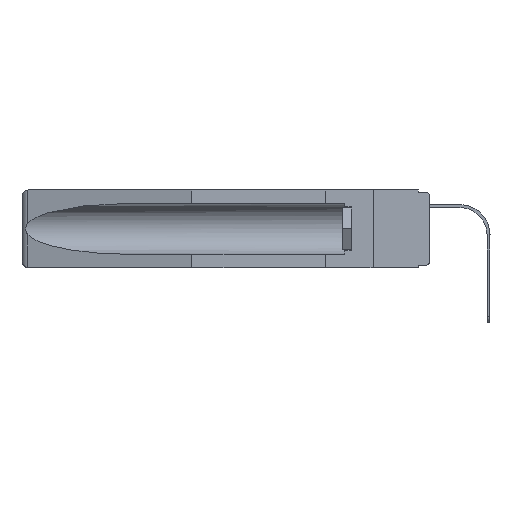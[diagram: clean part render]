
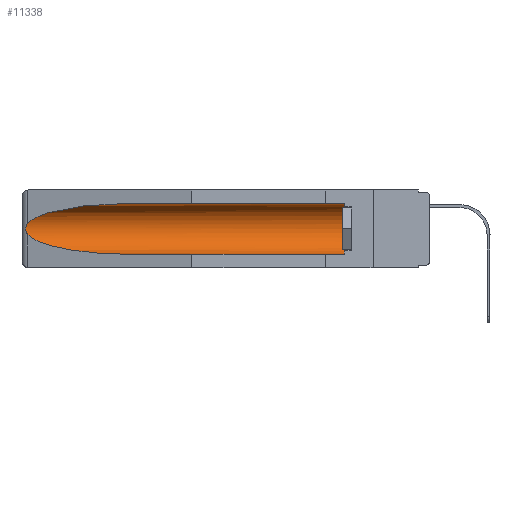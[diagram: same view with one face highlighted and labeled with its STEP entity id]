
A CAD part, left-side view. The second image highlights one B-rep face of the part: STEP entity #11338.
In plain terms, the highlighted cylindrical face has radius 2.857 mm (diameter 5.715 mm), a partial arc.
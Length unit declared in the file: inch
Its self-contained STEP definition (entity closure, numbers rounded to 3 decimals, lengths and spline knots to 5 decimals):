
#550 = EDGE_LOOP ( 'NONE', ( #24574, #18355, #9766, #16746, #15349, #6919 ) ) ;
#585 = CARTESIAN_POINT ( 'NONE',  ( 0.21114, 1.30732, -0.284 ) ) ;
#744 = DIRECTION ( 'NONE',  ( 0., 1., 0. ) ) ;
#991 = DIRECTION ( 'NONE',  ( 0., -1., 0. ) ) ;
#1263 = AXIS2_PLACEMENT_3D ( 'NONE', #24435, #22390, #2885 ) ;
#2885 = DIRECTION ( 'NONE',  ( 0., 0., 1. ) ) ;
#3160 = CARTESIAN_POINT ( 'NONE',  ( 0.2675, 1.53308, -0.17534 ) ) ;
#3287 = CARTESIAN_POINT ( 'NONE',  ( 0.26597, 1.5296, -0.19026 ) ) ;
#4566 = EDGE_CURVE ( 'NONE', #14290, #7133, #9843, .T. ) ;
#4671 = VERTEX_POINT ( 'NONE', #20564 ) ;
#5633 = CARTESIAN_POINT ( 'NONE',  ( 0.155, -0.30754, -0.059 ) ) ;
#6863 = AXIS2_PLACEMENT_3D ( 'NONE', #12802, #991, #18305 ) ;
#6919 = ORIENTED_EDGE ( 'NONE', *, *, #4566, .T. ) ;
#7133 = VERTEX_POINT ( 'NONE', #23824 ) ;
#7263 = EDGE_CURVE ( 'NONE', #15653, #7328, #10865, .T. ) ;
#7293 = EDGE_CURVE ( 'NONE', #15653, #14290, #20357, .T. ) ;
#7328 = VERTEX_POINT ( 'NONE', #12676 ) ;
#7773 = EDGE_CURVE ( 'NONE', #4671, #7328, #22846, .T. ) ;
#8536 = CARTESIAN_POINT ( 'NONE',  ( 0.26537, 1.52718, -0.19328 ) ) ;
#8577 = EDGE_CURVE ( 'NONE', #12557, #4671, #16978, .T. ) ;
#9313 = CARTESIAN_POINT ( 'NONE',  ( 0.2673, 1.5327, -0.16383 ) ) ;
#9766 = ORIENTED_EDGE ( 'NONE', *, *, #7773, .T. ) ;
#9843 = LINE ( 'NONE', #5633, #10423 ) ;
#9967 = DIRECTION ( 'NONE',  ( 0., 1., 0. ) ) ;
#10423 = VECTOR ( 'NONE', #9967, 39.37008 ) ;
#10459 = FACE_OUTER_BOUND ( 'NONE', #550, .T. ) ;
#10865 = LINE ( 'NONE', #16646, #22420 ) ;
#11338 = ADVANCED_FACE ( 'NONE', ( #10459 ), #16618, .F. ) ;
#11370 = CARTESIAN_POINT ( 'NONE',  ( 0.26537, 1.52718, -0.19328 ) ) ;
#12557 = VERTEX_POINT ( 'NONE', #24482 ) ;
#12676 = CARTESIAN_POINT ( 'NONE',  ( 0.155, 1.07973, -0.284 ) ) ;
#12802 = CARTESIAN_POINT ( 'NONE',  ( 0.155, 0.126, -0.1715 ) ) ;
#12920 = CARTESIAN_POINT ( 'NONE',  ( 0.2675, 1.53308, -0.16763 ) ) ;
#14290 = VERTEX_POINT ( 'NONE', #20853 ) ;
#14327 = CARTESIAN_POINT ( 'NONE',  ( 0.155, 1.07973, -0.284 ) ) ;
#14851 = CARTESIAN_POINT ( 'NONE',  ( 0.26654, 1.53092, -0.15636 ) ) ;
#15349 = ORIENTED_EDGE ( 'NONE', *, *, #7293, .T. ) ;
#15653 = VERTEX_POINT ( 'NONE', #22382 ) ;
#15775 = CARTESIAN_POINT ( 'NONE',  ( 0.21114, 1.30732, -0.059 ) ) ;
#16501 = EDGE_CURVE ( 'NONE', #7133, #12557, #17585, .T. ) ;
#16618 = CYLINDRICAL_SURFACE ( 'NONE', #1263, 0.1125 ) ;
#16646 = CARTESIAN_POINT ( 'NONE',  ( 0.155, -0.30754, -0.284 ) ) ;
#16746 = ORIENTED_EDGE ( 'NONE', *, *, #7263, .F. ) ;
#16884 = CARTESIAN_POINT ( 'NONE',  ( 0.2673, 1.53269, -0.17917 ) ) ;
#16978 = B_SPLINE_CURVE_WITH_KNOTS ( 'NONE', 3,
 ( #20725, #18921, #14851, #9313, #12920, #3160, #16884, #17147, #3287, #11370 ),
 .UNSPECIFIED., .F., .F.,
 ( 4, 2, 2, 2, 4 ),
 ( 0., 0.00029, 0.00058, 0.00087, 0.00117 ),
 .UNSPECIFIED. ) ;
#17147 = CARTESIAN_POINT ( 'NONE',  ( 0.26655, 1.53094, -0.18657 ) ) ;
#17585 =( BOUNDED_CURVE ( )  B_SPLINE_CURVE ( 3, ( #25017, #15775, #23336, #23092 ),
 .UNSPECIFIED., .F., .F. ) 
 B_SPLINE_CURVE_WITH_KNOTS ( ( 4, 4 ),
 ( 4.71239, 6.08839 ),
 .UNSPECIFIED. ) 
 CURVE ( )  GEOMETRIC_REPRESENTATION_ITEM ( )  RATIONAL_B_SPLINE_CURVE ( ( 1., 0.848, 0.848, 1. ) ) 
 REPRESENTATION_ITEM ( '' )  );
#18147 = CARTESIAN_POINT ( 'NONE',  ( 0.25451, 1.48313, -0.24835 ) ) ;
#18305 = DIRECTION ( 'NONE',  ( 0., 0., 1. ) ) ;
#18355 = ORIENTED_EDGE ( 'NONE', *, *, #8577, .T. ) ;
#18921 = CARTESIAN_POINT ( 'NONE',  ( 0.26597, 1.52961, -0.15275 ) ) ;
#20357 = CIRCLE ( 'NONE', #6863, 0.1125 ) ;
#20564 = CARTESIAN_POINT ( 'NONE',  ( 0.26537, 1.52718, -0.19328 ) ) ;
#20725 = CARTESIAN_POINT ( 'NONE',  ( 0.26537, 1.52718, -0.14972 ) ) ;
#20853 = CARTESIAN_POINT ( 'NONE',  ( 0.155, 0.126, -0.059 ) ) ;
#22382 = CARTESIAN_POINT ( 'NONE',  ( 0.155, 0.126, -0.284 ) ) ;
#22390 = DIRECTION ( 'NONE',  ( 0., 1., 0. ) ) ;
#22420 = VECTOR ( 'NONE', #744, 39.37008 ) ;
#22846 =( BOUNDED_CURVE ( )  B_SPLINE_CURVE ( 3, ( #8536, #18147, #585, #14327 ),
 .UNSPECIFIED., .F., .T. ) 
 B_SPLINE_CURVE_WITH_KNOTS ( ( 4, 4 ),
 ( 0.1948, 1.5708 ),
 .UNSPECIFIED. ) 
 CURVE ( )  GEOMETRIC_REPRESENTATION_ITEM ( )  RATIONAL_B_SPLINE_CURVE ( ( 1., 0.848, 0.848, 1. ) ) 
 REPRESENTATION_ITEM ( '' )  );
#23092 = CARTESIAN_POINT ( 'NONE',  ( 0.26537, 1.52718, -0.14972 ) ) ;
#23336 = CARTESIAN_POINT ( 'NONE',  ( 0.25451, 1.48313, -0.09465 ) ) ;
#23824 = CARTESIAN_POINT ( 'NONE',  ( 0.155, 1.07973, -0.059 ) ) ;
#24435 = CARTESIAN_POINT ( 'NONE',  ( 0.155, -0.30754, -0.1715 ) ) ;
#24482 = CARTESIAN_POINT ( 'NONE',  ( 0.26537, 1.52718, -0.14972 ) ) ;
#24574 = ORIENTED_EDGE ( 'NONE', *, *, #16501, .T. ) ;
#25017 = CARTESIAN_POINT ( 'NONE',  ( 0.155, 1.07973, -0.059 ) ) ;
